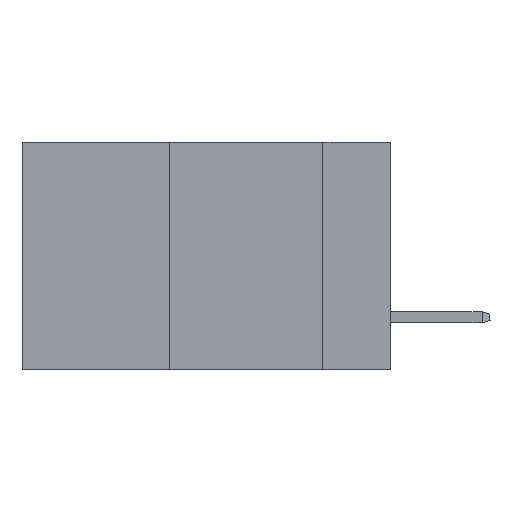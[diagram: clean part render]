
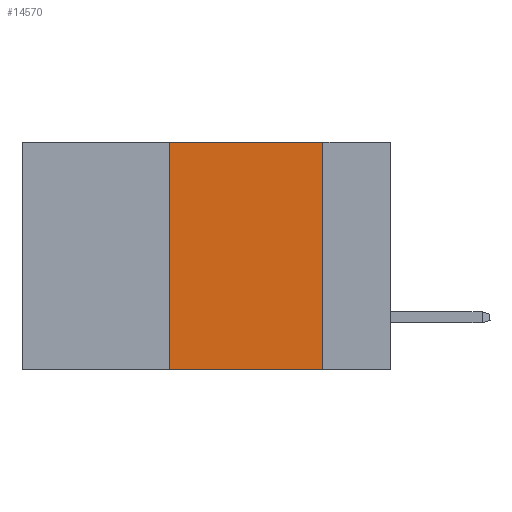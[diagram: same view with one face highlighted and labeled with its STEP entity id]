
A CAD part, left-side view. The second image highlights one B-rep face of the part: STEP entity #14570.
In plain terms, the highlighted planar face has unit normal (-1, 0, 0).
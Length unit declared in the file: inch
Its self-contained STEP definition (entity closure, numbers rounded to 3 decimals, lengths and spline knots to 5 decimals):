
#493 = FACE_OUTER_BOUND ( 'NONE', #26847, .T. ) ;
#704 = DIRECTION ( 'NONE',  ( 0., 0., -1. ) ) ;
#850 = CARTESIAN_POINT ( 'NONE',  ( 0., 0.6, 0. ) ) ;
#864 = AXIS2_PLACEMENT_3D ( 'NONE', #22040, #13992, #3626 ) ;
#1405 = LINE ( 'NONE', #13276, #24180 ) ;
#1928 = LINE ( 'NONE', #21036, #13289 ) ;
#1960 = ORIENTED_EDGE ( 'NONE', *, *, #12709, .F. ) ;
#3626 = DIRECTION ( 'NONE',  ( 0., 0., -1. ) ) ;
#4925 = EDGE_CURVE ( 'NONE', #32705, #8839, #1928, .T. ) ;
#6436 = ORIENTED_EDGE ( 'NONE', *, *, #4925, .F. ) ;
#7213 = CARTESIAN_POINT ( 'NONE',  ( 0., 0.11, -0.37 ) ) ;
#8839 = VERTEX_POINT ( 'NONE', #7213 ) ;
#10245 = VECTOR ( 'NONE', #22288, 39.37008 ) ;
#12709 = EDGE_CURVE ( 'NONE', #22112, #32705, #13095, .T. ) ;
#13095 = LINE ( 'NONE', #850, #24073 ) ;
#13276 = CARTESIAN_POINT ( 'NONE',  ( 0., 0.36, 0. ) ) ;
#13289 = VECTOR ( 'NONE', #704, 39.37008 ) ;
#13971 = CARTESIAN_POINT ( 'NONE',  ( 0., 0.36, 0. ) ) ;
#13992 = DIRECTION ( 'NONE',  ( 1., 0., 0. ) ) ;
#14452 = PLANE ( 'NONE',  #864 ) ;
#14570 = ADVANCED_FACE ( 'NONE', ( #493 ), #14452, .F. ) ;
#17761 = CARTESIAN_POINT ( 'NONE',  ( 0., 0.11, 0. ) ) ;
#19022 = DIRECTION ( 'NONE',  ( 0., -1., 0. ) ) ;
#19745 = EDGE_CURVE ( 'NONE', #30556, #8839, #31746, .T. ) ;
#19916 = CARTESIAN_POINT ( 'NONE',  ( 0., 0.6, -0.37 ) ) ;
#21036 = CARTESIAN_POINT ( 'NONE',  ( 0., 0.11, 0. ) ) ;
#21349 = CARTESIAN_POINT ( 'NONE',  ( 0., 0.36, -0.37 ) ) ;
#21840 = ORIENTED_EDGE ( 'NONE', *, *, #28398, .F. ) ;
#22040 = CARTESIAN_POINT ( 'NONE',  ( 0., 0.6, 0. ) ) ;
#22112 = VERTEX_POINT ( 'NONE', #13971 ) ;
#22288 = DIRECTION ( 'NONE',  ( 0., -1., 0. ) ) ;
#24073 = VECTOR ( 'NONE', #19022, 39.37008 ) ;
#24180 = VECTOR ( 'NONE', #25942, 39.37008 ) ;
#25942 = DIRECTION ( 'NONE',  ( 0., 0., 1. ) ) ;
#26847 = EDGE_LOOP ( 'NONE', ( #6436, #1960, #21840, #29516 ) ) ;
#28398 = EDGE_CURVE ( 'NONE', #30556, #22112, #1405, .T. ) ;
#29516 = ORIENTED_EDGE ( 'NONE', *, *, #19745, .T. ) ;
#30556 = VERTEX_POINT ( 'NONE', #21349 ) ;
#31746 = LINE ( 'NONE', #19916, #10245 ) ;
#32705 = VERTEX_POINT ( 'NONE', #17761 ) ;
